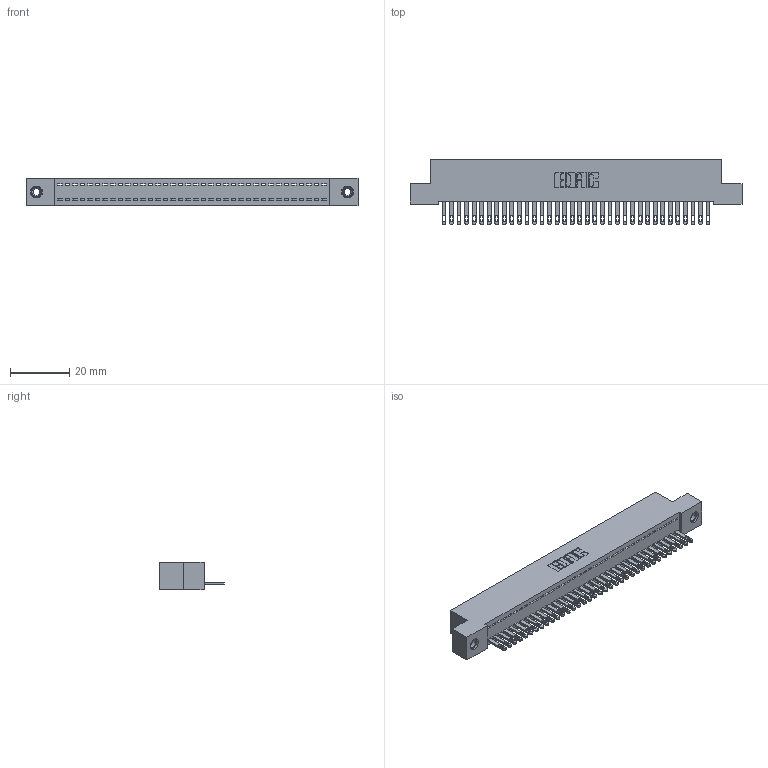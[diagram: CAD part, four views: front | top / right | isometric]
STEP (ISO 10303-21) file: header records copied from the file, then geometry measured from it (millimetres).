
FILE_DESCRIPTION (( 'STEP AP203' ), '1' );
FILE_NAME ('892-036-500-108.STEP', '2020-09-21T15:53:19', ( '' ), ( '' ), 'SwSTEP 2.0', 'SolidWorks 2020', '' );
FILE_SCHEMA (( 'CONFIG_CONTROL_DESIGN' ));
Length unit declared in the file: inch
Products named in the file (4): 345-292-001_345-293-100; 345-250-001_345-250-003-102; 842 Part_TI; 892-036-500-108
Assembly tree (39 placements, depth 2):
  892-036-500-108
    842 Part_TI
    345-292-001_345-293-100  x36
    345-250-001_345-250-003-102  x2
Bounding box: 111.76 x 21.85 x 9.4 mm (x, y, z)
Volume: 9793.6 mm3; surface area: 14358.1 mm2
Topology: 39 solids, 39 shells, 2114 faces, 6483 edges, 4314 vertices
Faces by surface type: plane 1394, cylinder 704, cone 12, torus 4
Entity records: 23768 total; most frequent: CARTESIAN_POINT 4081, ORIENTED_EDGE 4046, DIRECTION 3489, EDGE_CURVE 2023, VECTOR 1871, LINE 1871, VERTEX_POINT 1344, AXIS2_PLACEMENT_3D 809
